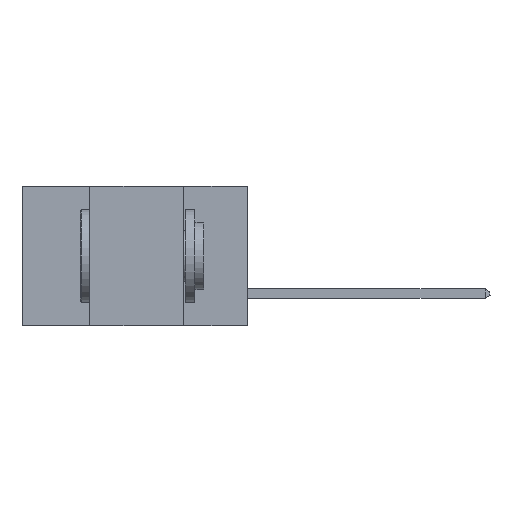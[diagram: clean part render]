
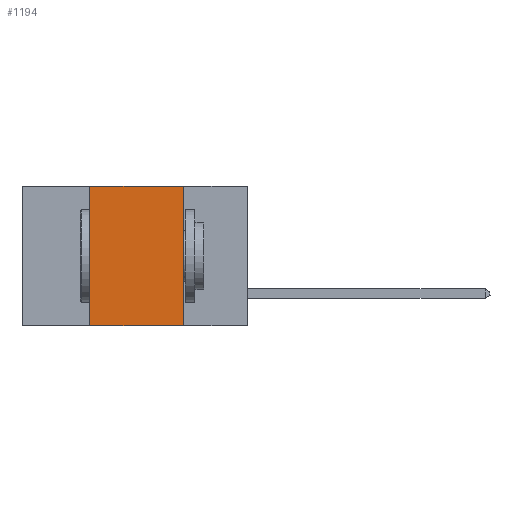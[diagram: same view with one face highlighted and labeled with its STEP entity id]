
A CAD part, left-side view. The second image highlights one B-rep face of the part: STEP entity #1194.
In plain terms, the highlighted planar face has unit normal (-1, 0, 0).
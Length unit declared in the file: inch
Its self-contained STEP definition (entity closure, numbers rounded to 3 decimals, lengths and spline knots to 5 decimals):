
#192 = VERTEX_POINT ( 'NONE', #6346 ) ;
#1171 = VERTEX_POINT ( 'NONE', #23939 ) ;
#1194 = ADVANCED_FACE ( 'NONE', ( #15414 ), #21390, .F. ) ;
#5611 = LINE ( 'NONE', #25535, #29572 ) ;
#6072 = CARTESIAN_POINT ( 'NONE',  ( 0., 0.17, -0.37 ) ) ;
#6267 = DIRECTION ( 'NONE',  ( 0., 0., 1. ) ) ;
#6346 = CARTESIAN_POINT ( 'NONE',  ( 0., 0.17, 0. ) ) ;
#6621 = VECTOR ( 'NONE', #10529, 39.37008 ) ;
#8378 = EDGE_CURVE ( 'NONE', #1171, #20079, #12148, .T. ) ;
#8444 = DIRECTION ( 'NONE',  ( 0., 0., -1. ) ) ;
#8633 = VERTEX_POINT ( 'NONE', #29799 ) ;
#10529 = DIRECTION ( 'NONE',  ( 0., -1., 0. ) ) ;
#11171 = VECTOR ( 'NONE', #28419, 39.37008 ) ;
#11549 = AXIS2_PLACEMENT_3D ( 'NONE', #21381, #24832, #8444 ) ;
#11553 = ORIENTED_EDGE ( 'NONE', *, *, #8378, .T. ) ;
#11841 = ORIENTED_EDGE ( 'NONE', *, *, #24003, .F. ) ;
#12148 = LINE ( 'NONE', #24450, #6621 ) ;
#13302 = ORIENTED_EDGE ( 'NONE', *, *, #29747, .F. ) ;
#14046 = LINE ( 'NONE', #27253, #14805 ) ;
#14742 = EDGE_LOOP ( 'NONE', ( #11841, #13302, #27129, #11553 ) ) ;
#14805 = VECTOR ( 'NONE', #6267, 39.37008 ) ;
#15414 = FACE_OUTER_BOUND ( 'NONE', #14742, .T. ) ;
#16359 = DIRECTION ( 'NONE',  ( 0., 0., -1. ) ) ;
#20079 = VERTEX_POINT ( 'NONE', #6072 ) ;
#21381 = CARTESIAN_POINT ( 'NONE',  ( 0., 0.6, 0. ) ) ;
#21390 = PLANE ( 'NONE',  #11549 ) ;
#23939 = CARTESIAN_POINT ( 'NONE',  ( 0., 0.42, -0.37 ) ) ;
#24003 = EDGE_CURVE ( 'NONE', #192, #20079, #5611, .T. ) ;
#24450 = CARTESIAN_POINT ( 'NONE',  ( 0., 0.6, -0.37 ) ) ;
#24832 = DIRECTION ( 'NONE',  ( 1., 0., 0. ) ) ;
#25535 = CARTESIAN_POINT ( 'NONE',  ( 0., 0.17, 0. ) ) ;
#26174 = CARTESIAN_POINT ( 'NONE',  ( 0., 0.6, 0. ) ) ;
#27129 = ORIENTED_EDGE ( 'NONE', *, *, #30069, .F. ) ;
#27253 = CARTESIAN_POINT ( 'NONE',  ( 0., 0.42, 0. ) ) ;
#28419 = DIRECTION ( 'NONE',  ( 0., -1., 0. ) ) ;
#29572 = VECTOR ( 'NONE', #16359, 39.37008 ) ;
#29575 = LINE ( 'NONE', #26174, #11171 ) ;
#29747 = EDGE_CURVE ( 'NONE', #8633, #192, #29575, .T. ) ;
#29799 = CARTESIAN_POINT ( 'NONE',  ( 0., 0.42, 0. ) ) ;
#30069 = EDGE_CURVE ( 'NONE', #1171, #8633, #14046, .T. ) ;
